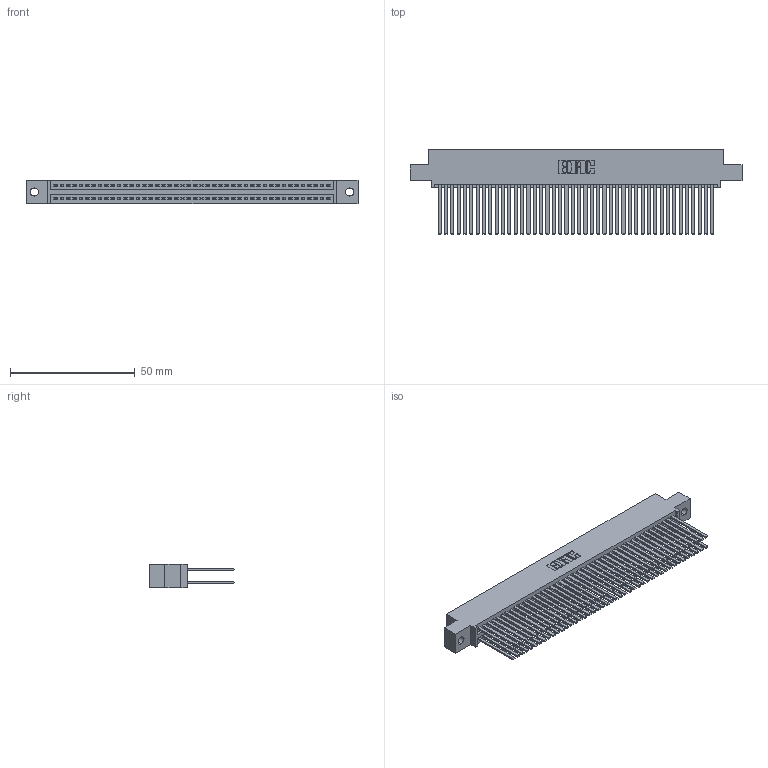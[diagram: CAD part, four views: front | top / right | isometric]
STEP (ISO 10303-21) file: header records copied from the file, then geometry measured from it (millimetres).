
FILE_DESCRIPTION (( 'STEP AP203' ), '1' );
FILE_NAME ('395-088-544-502.STEP', '2019-10-25T14:30:45', ( '' ), ( '' ), 'SwSTEP 2.0', 'SolidWorks 2016', '' );
FILE_SCHEMA (( 'CONFIG_CONTROL_DESIGN' ));
Length unit declared in the file: inch
Products named in the file (3): 345 Part_0.110 Offset - 0.128 Dia; 345-292-001_345-293-144; 395-088-544-502
Assembly tree (89 placements, depth 2):
  395-088-544-502
    345 Part_0.110 Offset - 0.128 Dia
    345-292-001_345-293-144  x88
Bounding box: 132.97 x 33.96 x 9.4 mm (x, y, z)
Volume: 14058.9 mm3; surface area: 24255.8 mm2
Topology: 89 solids, 89 shells, 4002 faces, 11881 edges, 7802 vertices
Faces by surface type: plane 2636, cylinder 1366
Entity records: 34205 total; most frequent: CARTESIAN_POINT 5732, ORIENTED_EDGE 5666, DIRECTION 5049, EDGE_CURVE 2833, LINE 2529, VECTOR 2529, VERTEX_POINT 1886, AXIS2_PLACEMENT_3D 1260
